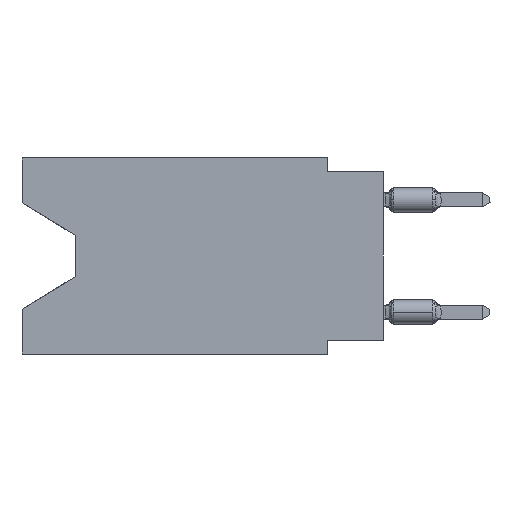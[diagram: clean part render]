
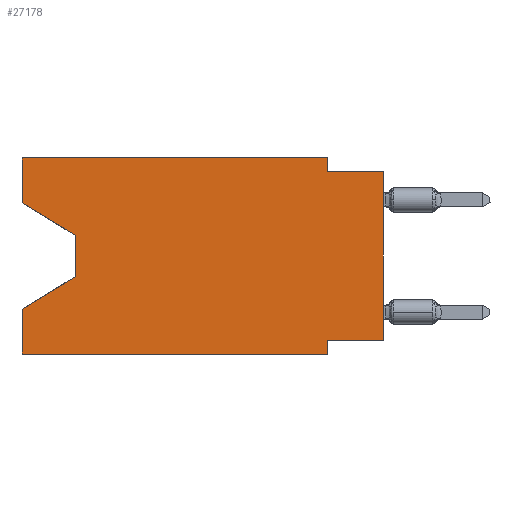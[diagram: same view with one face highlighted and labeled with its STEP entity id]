
A CAD part, left-side view. The second image highlights one B-rep face of the part: STEP entity #27178.
In plain terms, the highlighted planar face has unit normal (-1, 0, 0).
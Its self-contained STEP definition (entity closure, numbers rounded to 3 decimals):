
#489 = DIRECTION ( 'NONE',  ( 0., -1., 0. ) ) ;
#711 = VERTEX_POINT ( 'NONE', #28181 ) ;
#934 = LINE ( 'NONE', #13072, #16407 ) ;
#1153 = VERTEX_POINT ( 'NONE', #21778 ) ;
#1689 = EDGE_CURVE ( 'NONE', #14021, #7954, #12887, .T. ) ;
#2733 = EDGE_CURVE ( 'NONE', #14021, #42106, #3862, .T. ) ;
#2963 = PLANE ( 'NONE',  #45060 ) ;
#3862 = LINE ( 'NONE', #46308, #47852 ) ;
#4274 = LINE ( 'NONE', #35136, #36155 ) ;
#4472 = CARTESIAN_POINT ( 'NONE',  ( 0., 0., -8.255 ) ) ;
#5339 = LINE ( 'NONE', #47543, #38249 ) ;
#6934 = LINE ( 'NONE', #8689, #43186 ) ;
#7738 = LINE ( 'NONE', #12298, #10323 ) ;
#7954 = VERTEX_POINT ( 'NONE', #30881 ) ;
#8414 = EDGE_CURVE ( 'NONE', #36822, #1153, #7738, .T. ) ;
#8689 = CARTESIAN_POINT ( 'NONE',  ( 0., 2.54, 0. ) ) ;
#8856 = DIRECTION ( 'NONE',  ( 0., 0., -1. ) ) ;
#8965 = VERTEX_POINT ( 'NONE', #11752 ) ;
#10323 = VECTOR ( 'NONE', #23178, 1000. ) ;
#10410 = VERTEX_POINT ( 'NONE', #40803 ) ;
#10709 = CARTESIAN_POINT ( 'NONE',  ( 0., 0., -0.635 ) ) ;
#10979 = LINE ( 'NONE', #48886, #23151 ) ;
#11212 = DIRECTION ( 'NONE',  ( 0., -1., 0. ) ) ;
#11752 = CARTESIAN_POINT ( 'NONE',  ( 0., 16.383, -2.038 ) ) ;
#11920 = CARTESIAN_POINT ( 'NONE',  ( 0., 2.54, -0.635 ) ) ;
#12298 = CARTESIAN_POINT ( 'NONE',  ( 0., 13.97, -5.385 ) ) ;
#12887 = LINE ( 'NONE', #40423, #34086 ) ;
#13072 = CARTESIAN_POINT ( 'NONE',  ( 0., 2.54, -8.89 ) ) ;
#14021 = VERTEX_POINT ( 'NONE', #4472 ) ;
#14114 = DIRECTION ( 'NONE',  ( 1., 0., 0. ) ) ;
#14480 = ORIENTED_EDGE ( 'NONE', *, *, #33395, .F. ) ;
#14807 = ORIENTED_EDGE ( 'NONE', *, *, #22997, .F. ) ;
#15203 = VECTOR ( 'NONE', #11212, 1000. ) ;
#15373 = ORIENTED_EDGE ( 'NONE', *, *, #8414, .T. ) ;
#16407 = VECTOR ( 'NONE', #28509, 1000. ) ;
#16682 = DIRECTION ( 'NONE',  ( 0., 0., 1. ) ) ;
#16842 = VECTOR ( 'NONE', #22225, 1000. ) ;
#17132 = EDGE_CURVE ( 'NONE', #20243, #10410, #4274, .T. ) ;
#17910 = DIRECTION ( 'NONE',  ( 0., 0., -1. ) ) ;
#17957 = VERTEX_POINT ( 'NONE', #20094 ) ;
#19114 = ORIENTED_EDGE ( 'NONE', *, *, #23282, .F. ) ;
#20094 = CARTESIAN_POINT ( 'NONE',  ( 0., 16.383, 0. ) ) ;
#20243 = VERTEX_POINT ( 'NONE', #25287 ) ;
#21148 = EDGE_CURVE ( 'NONE', #8965, #17957, #10979, .T. ) ;
#21623 = ORIENTED_EDGE ( 'NONE', *, *, #1689, .T. ) ;
#21689 = VERTEX_POINT ( 'NONE', #11920 ) ;
#21778 = CARTESIAN_POINT ( 'NONE',  ( 0., 16.383, -6.852 ) ) ;
#22225 = DIRECTION ( 'NONE',  ( 0., 0., 1. ) ) ;
#22997 = EDGE_CURVE ( 'NONE', #21689, #7954, #30440, .T. ) ;
#23151 = VECTOR ( 'NONE', #29717, 1000. ) ;
#23178 = DIRECTION ( 'NONE',  ( 0., 0.855, -0.519 ) ) ;
#23252 = CARTESIAN_POINT ( 'NONE',  ( 0., 2.54, -8.255 ) ) ;
#23282 = EDGE_CURVE ( 'NONE', #20243, #1153, #49241, .T. ) ;
#23702 = DIRECTION ( 'NONE',  ( 0., -1., 0. ) ) ;
#23887 = EDGE_LOOP ( 'NONE', ( #49438, #25139, #15373, #19114, #36448, #14480, #25263, #21623, #14807, #39186, #30001, #24270 ) ) ;
#24270 = ORIENTED_EDGE ( 'NONE', *, *, #21148, .F. ) ;
#24963 = CARTESIAN_POINT ( 'NONE',  ( 0., 13.97, -5.385 ) ) ;
#25139 = ORIENTED_EDGE ( 'NONE', *, *, #49901, .T. ) ;
#25263 = ORIENTED_EDGE ( 'NONE', *, *, #2733, .F. ) ;
#25287 = CARTESIAN_POINT ( 'NONE',  ( 0., 16.383, -8.89 ) ) ;
#25986 = CARTESIAN_POINT ( 'NONE',  ( 0., 16.383, 0. ) ) ;
#27178 = ADVANCED_FACE ( 'NONE', ( #41644 ), #2963, .F. ) ;
#28006 = LINE ( 'NONE', #31297, #30267 ) ;
#28181 = CARTESIAN_POINT ( 'NONE',  ( 0., 13.97, -3.505 ) ) ;
#28509 = DIRECTION ( 'NONE',  ( 0., 0., -1. ) ) ;
#28566 = LINE ( 'NONE', #43470, #45196 ) ;
#29717 = DIRECTION ( 'NONE',  ( 0., 0., 1. ) ) ;
#30001 = ORIENTED_EDGE ( 'NONE', *, *, #43761, .F. ) ;
#30267 = VECTOR ( 'NONE', #23702, 1000. ) ;
#30440 = LINE ( 'NONE', #10709, #15203 ) ;
#30881 = CARTESIAN_POINT ( 'NONE',  ( 0., 0., -0.635 ) ) ;
#31297 = CARTESIAN_POINT ( 'NONE',  ( 0., 16.383, 0. ) ) ;
#33395 = EDGE_CURVE ( 'NONE', #42106, #10410, #934, .T. ) ;
#34086 = VECTOR ( 'NONE', #16682, 1000. ) ;
#35136 = CARTESIAN_POINT ( 'NONE',  ( 0., 16.383, -8.89 ) ) ;
#35450 = DIRECTION ( 'NONE',  ( 0., -0.855, -0.519 ) ) ;
#36155 = VECTOR ( 'NONE', #489, 1000. ) ;
#36448 = ORIENTED_EDGE ( 'NONE', *, *, #17132, .T. ) ;
#36822 = VERTEX_POINT ( 'NONE', #24963 ) ;
#38249 = VECTOR ( 'NONE', #35450, 1000. ) ;
#39186 = ORIENTED_EDGE ( 'NONE', *, *, #41209, .F. ) ;
#40423 = CARTESIAN_POINT ( 'NONE',  ( 0., 0., 0. ) ) ;
#40685 = CARTESIAN_POINT ( 'NONE',  ( 0., 16.383, 0. ) ) ;
#40803 = CARTESIAN_POINT ( 'NONE',  ( 0., 2.54, -8.89 ) ) ;
#41209 = EDGE_CURVE ( 'NONE', #44748, #21689, #6934, .T. ) ;
#41644 = FACE_OUTER_BOUND ( 'NONE', #23887, .T. ) ;
#42106 = VERTEX_POINT ( 'NONE', #23252 ) ;
#42800 = DIRECTION ( 'NONE',  ( 0., 1., 0. ) ) ;
#43186 = VECTOR ( 'NONE', #47072, 1000. ) ;
#43220 = CARTESIAN_POINT ( 'NONE',  ( 0., 2.54, 0. ) ) ;
#43470 = CARTESIAN_POINT ( 'NONE',  ( 0., 13.97, -3.505 ) ) ;
#43761 = EDGE_CURVE ( 'NONE', #17957, #44748, #28006, .T. ) ;
#44748 = VERTEX_POINT ( 'NONE', #43220 ) ;
#45060 = AXIS2_PLACEMENT_3D ( 'NONE', #25986, #14114, #17910 ) ;
#45196 = VECTOR ( 'NONE', #8856, 1000. ) ;
#46308 = CARTESIAN_POINT ( 'NONE',  ( 0., 0., -8.255 ) ) ;
#47072 = DIRECTION ( 'NONE',  ( 0., 0., -1. ) ) ;
#47543 = CARTESIAN_POINT ( 'NONE',  ( 0., 16.383, -2.038 ) ) ;
#47852 = VECTOR ( 'NONE', #42800, 1000. ) ;
#48275 = EDGE_CURVE ( 'NONE', #8965, #711, #5339, .T. ) ;
#48886 = CARTESIAN_POINT ( 'NONE',  ( 0., 16.383, 0. ) ) ;
#49241 = LINE ( 'NONE', #40685, #16842 ) ;
#49438 = ORIENTED_EDGE ( 'NONE', *, *, #48275, .T. ) ;
#49901 = EDGE_CURVE ( 'NONE', #711, #36822, #28566, .T. ) ;
